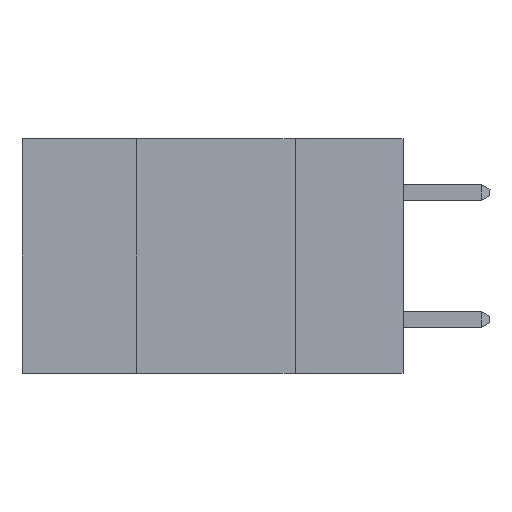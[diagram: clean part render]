
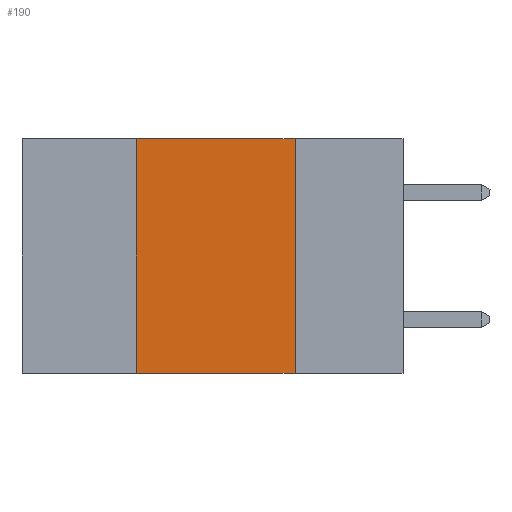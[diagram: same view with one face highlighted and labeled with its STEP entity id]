
A CAD part, left-side view. The second image highlights one B-rep face of the part: STEP entity #190.
In plain terms, the highlighted planar face has unit normal (-1, 0, 0).
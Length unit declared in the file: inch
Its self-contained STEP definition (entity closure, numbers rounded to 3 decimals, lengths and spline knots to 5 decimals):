
#54 = EDGE_CURVE ( 'NONE', #7979, #9177, #10021, .T. ) ;
#190 = ADVANCED_FACE ( 'NONE', ( #4995 ), #6074, .F. ) ;
#350 = VERTEX_POINT ( 'NONE', #1480 ) ;
#1011 = LINE ( 'NONE', #9530, #3366 ) ;
#1480 = CARTESIAN_POINT ( 'NONE',  ( 0., 0.17, 0. ) ) ;
#1995 = EDGE_LOOP ( 'NONE', ( #9405, #5353, #6027, #7526 ) ) ;
#2756 = DIRECTION ( 'NONE',  ( 0., 0., 1. ) ) ;
#2847 = VECTOR ( 'NONE', #8401, 39.37008 ) ;
#3366 = VECTOR ( 'NONE', #8052, 39.37008 ) ;
#4263 = DIRECTION ( 'NONE',  ( 0., 0., -1. ) ) ;
#4995 = FACE_OUTER_BOUND ( 'NONE', #1995, .T. ) ;
#5353 = ORIENTED_EDGE ( 'NONE', *, *, #6546, .F. ) ;
#5360 = VERTEX_POINT ( 'NONE', #7804 ) ;
#6027 = ORIENTED_EDGE ( 'NONE', *, *, #7005, .F. ) ;
#6074 = PLANE ( 'NONE',  #8682 ) ;
#6447 = CARTESIAN_POINT ( 'NONE',  ( 0., 0.6, -0.37 ) ) ;
#6546 = EDGE_CURVE ( 'NONE', #5360, #350, #8943, .T. ) ;
#6684 = DIRECTION ( 'NONE',  ( 1., 0., 0. ) ) ;
#6798 = VECTOR ( 'NONE', #9341, 39.37008 ) ;
#7005 = EDGE_CURVE ( 'NONE', #7979, #5360, #8836, .T. ) ;
#7055 = CARTESIAN_POINT ( 'NONE',  ( 0., 0.17, -0.37 ) ) ;
#7061 = VECTOR ( 'NONE', #2756, 39.37008 ) ;
#7116 = CARTESIAN_POINT ( 'NONE',  ( 0., 0.42, -0.37 ) ) ;
#7356 = CARTESIAN_POINT ( 'NONE',  ( 0., 0.42, 0. ) ) ;
#7509 = EDGE_CURVE ( 'NONE', #350, #9177, #1011, .T. ) ;
#7526 = ORIENTED_EDGE ( 'NONE', *, *, #54, .T. ) ;
#7623 = CARTESIAN_POINT ( 'NONE',  ( 0., 0.6, 0. ) ) ;
#7804 = CARTESIAN_POINT ( 'NONE',  ( 0., 0.42, 0. ) ) ;
#7979 = VERTEX_POINT ( 'NONE', #7116 ) ;
#8052 = DIRECTION ( 'NONE',  ( 0., 0., -1. ) ) ;
#8401 = DIRECTION ( 'NONE',  ( 0., -1., 0. ) ) ;
#8682 = AXIS2_PLACEMENT_3D ( 'NONE', #10314, #6684, #4263 ) ;
#8836 = LINE ( 'NONE', #7356, #7061 ) ;
#8943 = LINE ( 'NONE', #7623, #2847 ) ;
#9177 = VERTEX_POINT ( 'NONE', #7055 ) ;
#9341 = DIRECTION ( 'NONE',  ( 0., -1., 0. ) ) ;
#9405 = ORIENTED_EDGE ( 'NONE', *, *, #7509, .F. ) ;
#9530 = CARTESIAN_POINT ( 'NONE',  ( 0., 0.17, 0. ) ) ;
#10021 = LINE ( 'NONE', #6447, #6798 ) ;
#10314 = CARTESIAN_POINT ( 'NONE',  ( 0., 0.6, 0. ) ) ;
